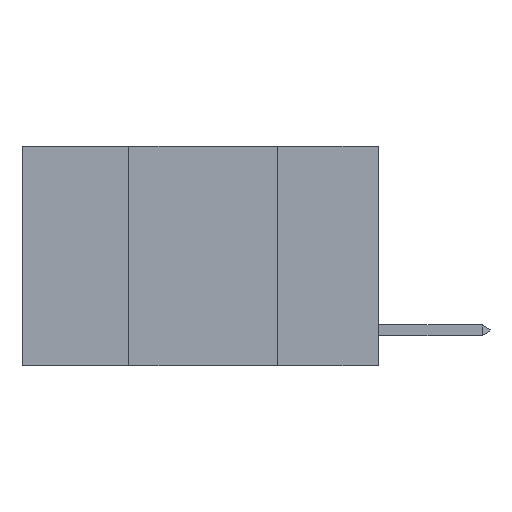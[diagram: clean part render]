
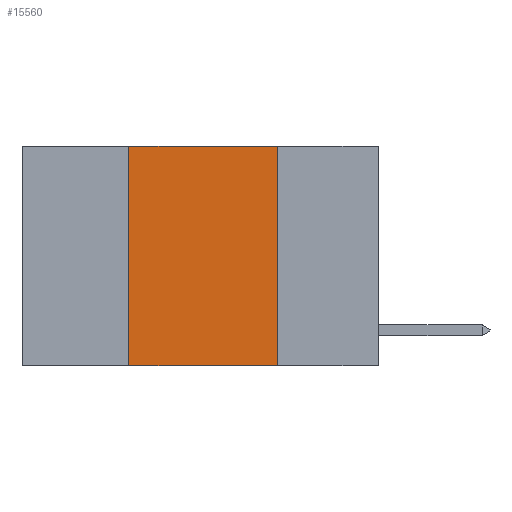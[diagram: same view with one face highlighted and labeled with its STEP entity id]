
A CAD part, left-side view. The second image highlights one B-rep face of the part: STEP entity #15560.
In plain terms, the highlighted planar face has unit normal (-1, 0, 0).
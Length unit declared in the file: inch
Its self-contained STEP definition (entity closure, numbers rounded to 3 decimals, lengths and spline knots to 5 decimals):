
#131 = DIRECTION ( 'NONE',  ( 0., 0., -1. ) ) ;
#156 = VECTOR ( 'NONE', #131, 39.37008 ) ;
#434 = EDGE_CURVE ( 'NONE', #5979, #2626, #12504, .T. ) ;
#594 = VERTEX_POINT ( 'NONE', #5645 ) ;
#625 = EDGE_CURVE ( 'NONE', #594, #6417, #5373, .T. ) ;
#879 = DIRECTION ( 'NONE',  ( 0., 0., 1. ) ) ;
#1732 = CARTESIAN_POINT ( 'NONE',  ( 0., 0.6, 0. ) ) ;
#2377 = EDGE_CURVE ( 'NONE', #594, #5979, #14333, .T. ) ;
#2626 = VERTEX_POINT ( 'NONE', #15115 ) ;
#3391 = CARTESIAN_POINT ( 'NONE',  ( 0., 0.6, -0.37 ) ) ;
#4123 = FACE_OUTER_BOUND ( 'NONE', #12524, .T. ) ;
#5373 = LINE ( 'NONE', #3391, #14367 ) ;
#5645 = CARTESIAN_POINT ( 'NONE',  ( 0., 0.42, -0.37 ) ) ;
#5727 = CARTESIAN_POINT ( 'NONE',  ( 0., 0.42, 0. ) ) ;
#5979 = VERTEX_POINT ( 'NONE', #7410 ) ;
#6203 = ORIENTED_EDGE ( 'NONE', *, *, #625, .T. ) ;
#6410 = DIRECTION ( 'NONE',  ( 1., 0., 0. ) ) ;
#6417 = VERTEX_POINT ( 'NONE', #14961 ) ;
#7410 = CARTESIAN_POINT ( 'NONE',  ( 0., 0.42, 0. ) ) ;
#7685 = DIRECTION ( 'NONE',  ( 0., -1., 0. ) ) ;
#8595 = ORIENTED_EDGE ( 'NONE', *, *, #13929, .F. ) ;
#8883 = CARTESIAN_POINT ( 'NONE',  ( 0., 0.6, 0. ) ) ;
#9115 = DIRECTION ( 'NONE',  ( 0., 0., -1. ) ) ;
#11194 = VECTOR ( 'NONE', #7685, 39.37008 ) ;
#11223 = CARTESIAN_POINT ( 'NONE',  ( 0., 0.17, 0. ) ) ;
#12052 = VECTOR ( 'NONE', #879, 39.37008 ) ;
#12504 = LINE ( 'NONE', #8883, #11194 ) ;
#12524 = EDGE_LOOP ( 'NONE', ( #8595, #13520, #12998, #6203 ) ) ;
#12998 = ORIENTED_EDGE ( 'NONE', *, *, #2377, .F. ) ;
#13520 = ORIENTED_EDGE ( 'NONE', *, *, #434, .F. ) ;
#13929 = EDGE_CURVE ( 'NONE', #2626, #6417, #14334, .T. ) ;
#13953 = PLANE ( 'NONE',  #14703 ) ;
#14333 = LINE ( 'NONE', #5727, #12052 ) ;
#14334 = LINE ( 'NONE', #11223, #156 ) ;
#14367 = VECTOR ( 'NONE', #14382, 39.37008 ) ;
#14382 = DIRECTION ( 'NONE',  ( 0., -1., 0. ) ) ;
#14703 = AXIS2_PLACEMENT_3D ( 'NONE', #1732, #6410, #9115 ) ;
#14961 = CARTESIAN_POINT ( 'NONE',  ( 0., 0.17, -0.37 ) ) ;
#15115 = CARTESIAN_POINT ( 'NONE',  ( 0., 0.17, 0. ) ) ;
#15560 = ADVANCED_FACE ( 'NONE', ( #4123 ), #13953, .F. ) ;
